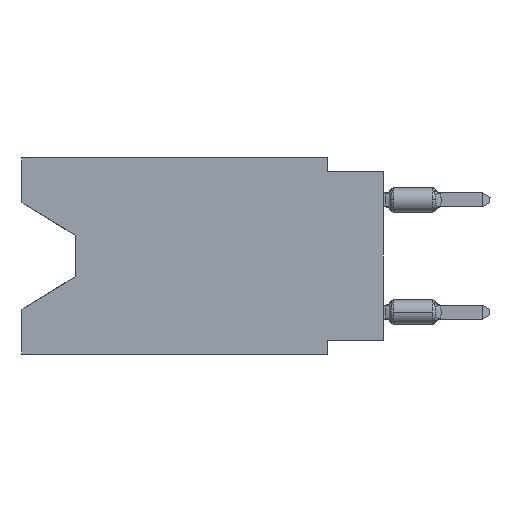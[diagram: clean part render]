
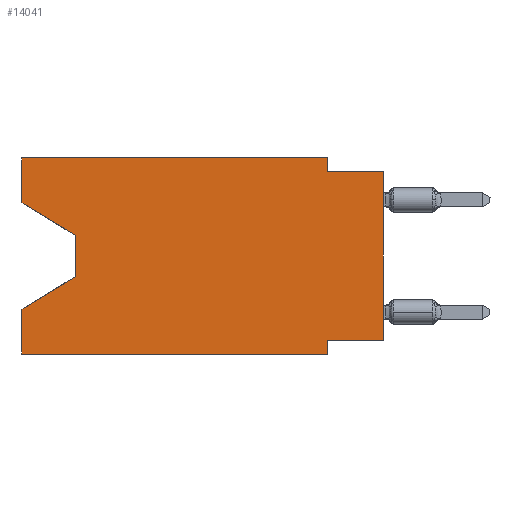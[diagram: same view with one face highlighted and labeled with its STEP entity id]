
A CAD part, left-side view. The second image highlights one B-rep face of the part: STEP entity #14041.
In plain terms, the highlighted planar face has unit normal (-1, 0, 0).
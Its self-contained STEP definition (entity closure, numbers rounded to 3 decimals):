
#419 = LINE ( 'NONE', #21339, #10931 ) ;
#574 = ORIENTED_EDGE ( 'NONE', *, *, #22529, .T. ) ;
#1274 = EDGE_CURVE ( 'NONE', #26973, #16873, #7215, .T. ) ;
#2139 = DIRECTION ( 'NONE',  ( 0., 0., 1. ) ) ;
#2313 = CARTESIAN_POINT ( 'NONE',  ( 0., 16.383, -2.038 ) ) ;
#2805 = VECTOR ( 'NONE', #30007, 1000. ) ;
#3679 = ORIENTED_EDGE ( 'NONE', *, *, #5902, .F. ) ;
#4150 = DIRECTION ( 'NONE',  ( 0., 0., -1. ) ) ;
#4160 = CARTESIAN_POINT ( 'NONE',  ( 0., 16.383, 0. ) ) ;
#4261 = VECTOR ( 'NONE', #6125, 1000. ) ;
#4690 = CARTESIAN_POINT ( 'NONE',  ( 0., 2.54, 0. ) ) ;
#4817 = PLANE ( 'NONE',  #16261 ) ;
#5203 = LINE ( 'NONE', #23563, #27478 ) ;
#5337 = ORIENTED_EDGE ( 'NONE', *, *, #21189, .F. ) ;
#5568 = ORIENTED_EDGE ( 'NONE', *, *, #11144, .F. ) ;
#5646 = CARTESIAN_POINT ( 'NONE',  ( 0., 13.97, -5.385 ) ) ;
#5902 = EDGE_CURVE ( 'NONE', #11269, #9514, #8774, .T. ) ;
#6046 = CARTESIAN_POINT ( 'NONE',  ( 0., 13.97, -3.505 ) ) ;
#6125 = DIRECTION ( 'NONE',  ( 0., 0., -1. ) ) ;
#6691 = LINE ( 'NONE', #17052, #33501 ) ;
#7215 = LINE ( 'NONE', #17585, #30445 ) ;
#7729 = ORIENTED_EDGE ( 'NONE', *, *, #30183, .T. ) ;
#8241 = ORIENTED_EDGE ( 'NONE', *, *, #1274, .T. ) ;
#8774 = LINE ( 'NONE', #4160, #22138 ) ;
#8830 = LINE ( 'NONE', #29558, #20907 ) ;
#8853 = LINE ( 'NONE', #29419, #4261 ) ;
#9514 = VERTEX_POINT ( 'NONE', #11914 ) ;
#9966 = CARTESIAN_POINT ( 'NONE',  ( 0., 2.54, -8.255 ) ) ;
#10295 = LINE ( 'NONE', #2313, #30841 ) ;
#10779 = LINE ( 'NONE', #29133, #29330 ) ;
#10931 = VECTOR ( 'NONE', #18779, 1000. ) ;
#11144 = EDGE_CURVE ( 'NONE', #15514, #16873, #8853, .T. ) ;
#11269 = VERTEX_POINT ( 'NONE', #23743 ) ;
#11282 = ORIENTED_EDGE ( 'NONE', *, *, #27986, .F. ) ;
#11360 = VERTEX_POINT ( 'NONE', #30031 ) ;
#11684 = ORIENTED_EDGE ( 'NONE', *, *, #14840, .T. ) ;
#11914 = CARTESIAN_POINT ( 'NONE',  ( 0., 2.54, 0. ) ) ;
#12123 = DIRECTION ( 'NONE',  ( 1., 0., 0. ) ) ;
#12435 = ORIENTED_EDGE ( 'NONE', *, *, #33428, .F. ) ;
#13031 = EDGE_CURVE ( 'NONE', #30624, #28409, #17140, .T. ) ;
#13740 = VERTEX_POINT ( 'NONE', #6046 ) ;
#14041 = ADVANCED_FACE ( 'NONE', ( #25562 ), #4817, .F. ) ;
#14114 = EDGE_LOOP ( 'NONE', ( #11684, #7729, #574, #5337, #8241, #5568, #12435, #22486, #11282, #31399, #3679, #22831 ) ) ;
#14197 = DIRECTION ( 'NONE',  ( 0., -1., 0. ) ) ;
#14382 = CARTESIAN_POINT ( 'NONE',  ( 0., 0., -0.635 ) ) ;
#14840 = EDGE_CURVE ( 'NONE', #25958, #13740, #10295, .T. ) ;
#14930 = VECTOR ( 'NONE', #22889, 1000. ) ;
#15458 = CARTESIAN_POINT ( 'NONE',  ( 0., 16.383, -2.038 ) ) ;
#15514 = VERTEX_POINT ( 'NONE', #9966 ) ;
#16261 = AXIS2_PLACEMENT_3D ( 'NONE', #33048, #12123, #33378 ) ;
#16725 = EDGE_CURVE ( 'NONE', #25958, #11269, #5203, .T. ) ;
#16873 = VERTEX_POINT ( 'NONE', #21694 ) ;
#16984 = DIRECTION ( 'NONE',  ( 0., 0., 1. ) ) ;
#17052 = CARTESIAN_POINT ( 'NONE',  ( 0., 13.97, -3.505 ) ) ;
#17140 = LINE ( 'NONE', #19722, #24464 ) ;
#17585 = CARTESIAN_POINT ( 'NONE',  ( 0., 16.383, -8.89 ) ) ;
#18093 = VERTEX_POINT ( 'NONE', #26123 ) ;
#18779 = DIRECTION ( 'NONE',  ( 0., 0.855, -0.519 ) ) ;
#19722 = CARTESIAN_POINT ( 'NONE',  ( 0., 0., 0. ) ) ;
#20179 = DIRECTION ( 'NONE',  ( 0., -0.855, -0.519 ) ) ;
#20573 = CARTESIAN_POINT ( 'NONE',  ( 0., 0., -8.255 ) ) ;
#20907 = VECTOR ( 'NONE', #24468, 1000. ) ;
#21189 = EDGE_CURVE ( 'NONE', #26973, #11360, #10779, .T. ) ;
#21339 = CARTESIAN_POINT ( 'NONE',  ( 0., 13.97, -5.385 ) ) ;
#21694 = CARTESIAN_POINT ( 'NONE',  ( 0., 2.54, -8.89 ) ) ;
#22138 = VECTOR ( 'NONE', #14197, 1000. ) ;
#22486 = ORIENTED_EDGE ( 'NONE', *, *, #13031, .T. ) ;
#22529 = EDGE_CURVE ( 'NONE', #29060, #11360, #419, .T. ) ;
#22831 = ORIENTED_EDGE ( 'NONE', *, *, #16725, .F. ) ;
#22889 = DIRECTION ( 'NONE',  ( 0., 0., -1. ) ) ;
#23563 = CARTESIAN_POINT ( 'NONE',  ( 0., 16.383, 0. ) ) ;
#23743 = CARTESIAN_POINT ( 'NONE',  ( 0., 16.383, 0. ) ) ;
#24464 = VECTOR ( 'NONE', #16984, 1000. ) ;
#24468 = DIRECTION ( 'NONE',  ( 0., -1., 0. ) ) ;
#25562 = FACE_OUTER_BOUND ( 'NONE', #14114, .T. ) ;
#25633 = EDGE_CURVE ( 'NONE', #9514, #18093, #27979, .T. ) ;
#25958 = VERTEX_POINT ( 'NONE', #15458 ) ;
#26123 = CARTESIAN_POINT ( 'NONE',  ( 0., 2.54, -0.635 ) ) ;
#26973 = VERTEX_POINT ( 'NONE', #31711 ) ;
#27478 = VECTOR ( 'NONE', #2139, 1000. ) ;
#27605 = LINE ( 'NONE', #30159, #2805 ) ;
#27954 = DIRECTION ( 'NONE',  ( 0., -1., 0. ) ) ;
#27979 = LINE ( 'NONE', #4690, #14930 ) ;
#27986 = EDGE_CURVE ( 'NONE', #18093, #28409, #8830, .T. ) ;
#28409 = VERTEX_POINT ( 'NONE', #14382 ) ;
#29060 = VERTEX_POINT ( 'NONE', #5646 ) ;
#29133 = CARTESIAN_POINT ( 'NONE',  ( 0., 16.383, 0. ) ) ;
#29330 = VECTOR ( 'NONE', #31019, 1000. ) ;
#29419 = CARTESIAN_POINT ( 'NONE',  ( 0., 2.54, -8.89 ) ) ;
#29558 = CARTESIAN_POINT ( 'NONE',  ( 0., 0., -0.635 ) ) ;
#30007 = DIRECTION ( 'NONE',  ( 0., 1., 0. ) ) ;
#30031 = CARTESIAN_POINT ( 'NONE',  ( 0., 16.383, -6.852 ) ) ;
#30159 = CARTESIAN_POINT ( 'NONE',  ( 0., 0., -8.255 ) ) ;
#30183 = EDGE_CURVE ( 'NONE', #13740, #29060, #6691, .T. ) ;
#30445 = VECTOR ( 'NONE', #27954, 1000. ) ;
#30624 = VERTEX_POINT ( 'NONE', #20573 ) ;
#30841 = VECTOR ( 'NONE', #20179, 1000. ) ;
#31019 = DIRECTION ( 'NONE',  ( 0., 0., 1. ) ) ;
#31399 = ORIENTED_EDGE ( 'NONE', *, *, #25633, .F. ) ;
#31711 = CARTESIAN_POINT ( 'NONE',  ( 0., 16.383, -8.89 ) ) ;
#33048 = CARTESIAN_POINT ( 'NONE',  ( 0., 16.383, 0. ) ) ;
#33378 = DIRECTION ( 'NONE',  ( 0., 0., -1. ) ) ;
#33428 = EDGE_CURVE ( 'NONE', #30624, #15514, #27605, .T. ) ;
#33501 = VECTOR ( 'NONE', #4150, 1000. ) ;
